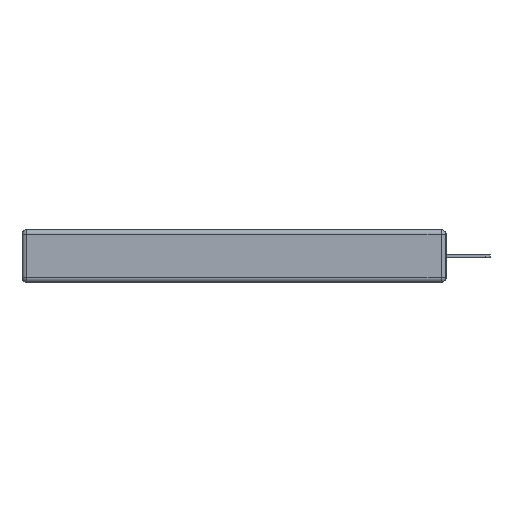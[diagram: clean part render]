
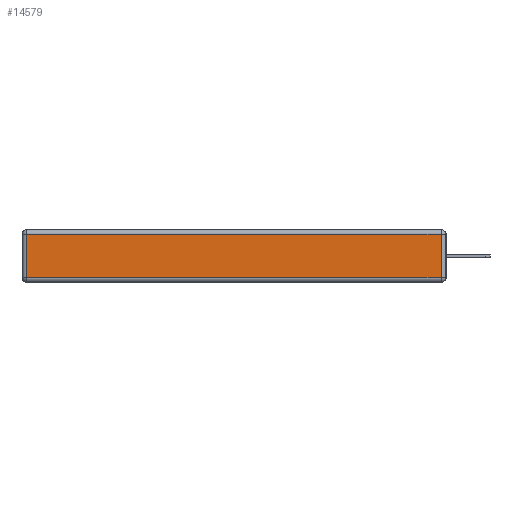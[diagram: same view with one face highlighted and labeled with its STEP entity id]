
A CAD part, left-side view. The second image highlights one B-rep face of the part: STEP entity #14579.
In plain terms, the highlighted planar face has unit normal (-1, 0, 0).
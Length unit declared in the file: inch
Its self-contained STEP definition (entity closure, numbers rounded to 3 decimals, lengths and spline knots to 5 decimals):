
#205 = EDGE_CURVE ( 'NONE', #25076, #23384, #12023, .T. ) ;
#2086 = PLANE ( 'NONE',  #3743 ) ;
#2650 = EDGE_CURVE ( 'NONE', #24253, #25076, #12131, .T. ) ;
#3333 = ORIENTED_EDGE ( 'NONE', *, *, #2650, .T. ) ;
#3390 = DIRECTION ( 'NONE',  ( 0., 1., 0. ) ) ;
#3743 = AXIS2_PLACEMENT_3D ( 'NONE', #14650, #6003, #27536 ) ;
#3780 = VERTEX_POINT ( 'NONE', #21930 ) ;
#4034 = DIRECTION ( 'NONE',  ( 0., -1., 0. ) ) ;
#5566 = EDGE_LOOP ( 'NONE', ( #3333, #24449, #9950, #18231 ) ) ;
#5603 = DIRECTION ( 'NONE',  ( 0., 0., 1. ) ) ;
#6003 = DIRECTION ( 'NONE',  ( -1., 0., 0. ) ) ;
#6079 = EDGE_CURVE ( 'NONE', #23384, #3780, #13571, .T. ) ;
#8328 = DIRECTION ( 'NONE',  ( 0., 0., -1. ) ) ;
#9950 = ORIENTED_EDGE ( 'NONE', *, *, #6079, .T. ) ;
#12023 = LINE ( 'NONE', #27009, #14371 ) ;
#12131 = LINE ( 'NONE', #27513, #13071 ) ;
#12860 = VECTOR ( 'NONE', #8328, 39.37008 ) ;
#13071 = VECTOR ( 'NONE', #4034, 39.37008 ) ;
#13571 = LINE ( 'NONE', #17940, #19246 ) ;
#14042 = CARTESIAN_POINT ( 'NONE',  ( 0., 0.03, -0.03 ) ) ;
#14371 = VECTOR ( 'NONE', #5603, 39.37008 ) ;
#14579 = ADVANCED_FACE ( 'NONE', ( #19002 ), #2086, .T. ) ;
#14650 = CARTESIAN_POINT ( 'NONE',  ( 0., 0., -0.343 ) ) ;
#17940 = CARTESIAN_POINT ( 'NONE',  ( 0., 2.75, -0.03 ) ) ;
#18066 = CARTESIAN_POINT ( 'NONE',  ( 0., 2.72, -0.313 ) ) ;
#18231 = ORIENTED_EDGE ( 'NONE', *, *, #19809, .T. ) ;
#18956 = LINE ( 'NONE', #27493, #12860 ) ;
#19002 = FACE_OUTER_BOUND ( 'NONE', #5566, .T. ) ;
#19246 = VECTOR ( 'NONE', #3390, 39.37008 ) ;
#19809 = EDGE_CURVE ( 'NONE', #3780, #24253, #18956, .T. ) ;
#21930 = CARTESIAN_POINT ( 'NONE',  ( 0., 2.72, -0.03 ) ) ;
#23384 = VERTEX_POINT ( 'NONE', #14042 ) ;
#24253 = VERTEX_POINT ( 'NONE', #18066 ) ;
#24449 = ORIENTED_EDGE ( 'NONE', *, *, #205, .T. ) ;
#25076 = VERTEX_POINT ( 'NONE', #26915 ) ;
#26915 = CARTESIAN_POINT ( 'NONE',  ( 0., 0.03, -0.313 ) ) ;
#27009 = CARTESIAN_POINT ( 'NONE',  ( 0., 0.03, -0.343 ) ) ;
#27493 = CARTESIAN_POINT ( 'NONE',  ( 0., 2.72, -0.343 ) ) ;
#27513 = CARTESIAN_POINT ( 'NONE',  ( 0., 0., -0.313 ) ) ;
#27536 = DIRECTION ( 'NONE',  ( 0., 0., 1. ) ) ;
